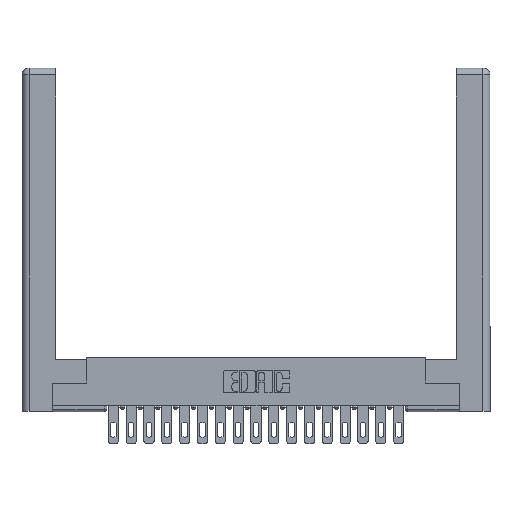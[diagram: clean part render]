
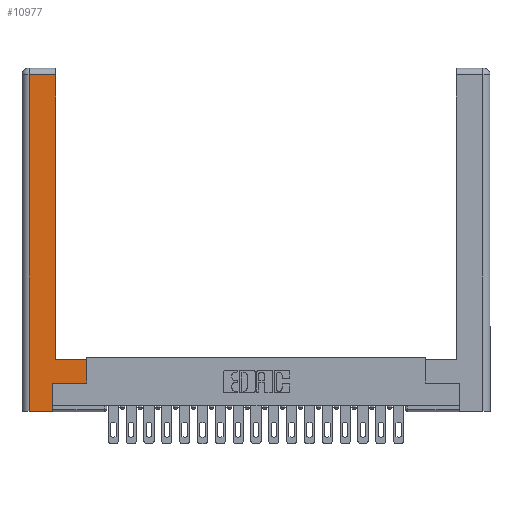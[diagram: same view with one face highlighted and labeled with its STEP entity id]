
A CAD part, top view. The second image highlights one B-rep face of the part: STEP entity #10977.
In plain terms, the highlighted planar face has unit normal (0, 0, 1).
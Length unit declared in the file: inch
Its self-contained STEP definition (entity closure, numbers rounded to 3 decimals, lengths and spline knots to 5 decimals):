
#130 = EDGE_CURVE ( 'NONE', #17198, #17549, #19335, .T. ) ;
#719 = PLANE ( 'NONE',  #18555 ) ;
#795 = ORIENTED_EDGE ( 'NONE', *, *, #10152, .T. ) ;
#1001 = ORIENTED_EDGE ( 'NONE', *, *, #14866, .T. ) ;
#1202 = ORIENTED_EDGE ( 'NONE', *, *, #11225, .T. ) ;
#1376 = CARTESIAN_POINT ( 'NONE',  ( 0.565, 0.245, 0. ) ) ;
#1582 = VERTEX_POINT ( 'NONE', #1671 ) ;
#1671 = CARTESIAN_POINT ( 'NONE',  ( 0.295, 2.94, 0. ) ) ;
#2708 = CARTESIAN_POINT ( 'NONE',  ( 0.265, 0.245, 0. ) ) ;
#3044 = EDGE_CURVE ( 'NONE', #17549, #8163, #11944, .T. ) ;
#3163 = EDGE_CURVE ( 'NONE', #14933, #9440, #14463, .T. ) ;
#3374 = ORIENTED_EDGE ( 'NONE', *, *, #130, .T. ) ;
#3509 = DIRECTION ( 'NONE',  ( 1., 0., 0. ) ) ;
#3822 = ORIENTED_EDGE ( 'NONE', *, *, #12952, .T. ) ;
#4591 = DIRECTION ( 'NONE',  ( 0., 1., 0. ) ) ;
#4656 = DIRECTION ( 'NONE',  ( 0., -1., 0. ) ) ;
#4859 = CARTESIAN_POINT ( 'NONE',  ( 0.0615, 0., 0. ) ) ;
#4863 = CARTESIAN_POINT ( 'NONE',  ( 0.265, 0., 0. ) ) ;
#5012 = CARTESIAN_POINT ( 'NONE',  ( 0.565, 0.45, 0. ) ) ;
#5196 = ORIENTED_EDGE ( 'NONE', *, *, #3044, .T. ) ;
#5393 = VECTOR ( 'NONE', #10994, 39.37008 ) ;
#5498 = CARTESIAN_POINT ( 'NONE',  ( 0., 0., 0. ) ) ;
#5504 = VECTOR ( 'NONE', #9365, 39.37008 ) ;
#6455 = EDGE_LOOP ( 'NONE', ( #795, #1202, #3822, #3374, #5196, #1001, #17080, #10570 ) ) ;
#6642 = DIRECTION ( 'NONE',  ( 0., 1., 0. ) ) ;
#6929 = DIRECTION ( 'NONE',  ( 0., 0., -1. ) ) ;
#7868 = CARTESIAN_POINT ( 'NONE',  ( 0.295, 3., 0. ) ) ;
#8163 = VERTEX_POINT ( 'NONE', #2708 ) ;
#9060 = CARTESIAN_POINT ( 'NONE',  ( 0.265, 0.245, 0. ) ) ;
#9365 = DIRECTION ( 'NONE',  ( 1., 0., 0. ) ) ;
#9440 = VERTEX_POINT ( 'NONE', #19036 ) ;
#9892 = EDGE_CURVE ( 'NONE', #9440, #15256, #20222, .T. ) ;
#10107 = CARTESIAN_POINT ( 'NONE',  ( 0.0615, 2.94, 0. ) ) ;
#10152 = EDGE_CURVE ( 'NONE', #15256, #1582, #18677, .T. ) ;
#10398 = VECTOR ( 'NONE', #3509, 39.37008 ) ;
#10570 = ORIENTED_EDGE ( 'NONE', *, *, #9892, .T. ) ;
#10977 = ADVANCED_FACE ( 'NONE', ( #11582 ), #719, .F. ) ;
#10994 = DIRECTION ( 'NONE',  ( -1., 0., 0. ) ) ;
#11125 = LINE ( 'NONE', #4859, #18955 ) ;
#11225 = EDGE_CURVE ( 'NONE', #1582, #20053, #15953, .T. ) ;
#11463 = CARTESIAN_POINT ( 'NONE',  ( 0.0615, 0., 0. ) ) ;
#11582 = FACE_OUTER_BOUND ( 'NONE', #6455, .T. ) ;
#11944 = LINE ( 'NONE', #9060, #19450 ) ;
#12004 = VECTOR ( 'NONE', #16057, 39.37008 ) ;
#12952 = EDGE_CURVE ( 'NONE', #20053, #17198, #11125, .T. ) ;
#13089 = VECTOR ( 'NONE', #6642, 39.37008 ) ;
#13216 = DIRECTION ( 'NONE',  ( -1., 0., 0. ) ) ;
#13477 = DIRECTION ( 'NONE',  ( 0., 1., 0. ) ) ;
#14275 = CARTESIAN_POINT ( 'NONE',  ( 0.565, 0.245, 0. ) ) ;
#14463 = LINE ( 'NONE', #5012, #13089 ) ;
#14707 = CARTESIAN_POINT ( 'NONE',  ( 0.0615, 2.94, 0. ) ) ;
#14866 = EDGE_CURVE ( 'NONE', #8163, #14933, #15520, .T. ) ;
#14933 = VERTEX_POINT ( 'NONE', #14275 ) ;
#15256 = VERTEX_POINT ( 'NONE', #19903 ) ;
#15520 = LINE ( 'NONE', #1376, #5504 ) ;
#15953 = LINE ( 'NONE', #14707, #12004 ) ;
#16057 = DIRECTION ( 'NONE',  ( -1., 0., 0. ) ) ;
#16344 = CARTESIAN_POINT ( 'NONE',  ( 0.265, 0., 0. ) ) ;
#17080 = ORIENTED_EDGE ( 'NONE', *, *, #3163, .T. ) ;
#17198 = VERTEX_POINT ( 'NONE', #11463 ) ;
#17222 = VECTOR ( 'NONE', #4591, 39.37008 ) ;
#17549 = VERTEX_POINT ( 'NONE', #4863 ) ;
#18555 = AXIS2_PLACEMENT_3D ( 'NONE', #5498, #6929, #13216 ) ;
#18677 = LINE ( 'NONE', #7868, #17222 ) ;
#18904 = CARTESIAN_POINT ( 'NONE',  ( 0.295, 0.45, 0. ) ) ;
#18955 = VECTOR ( 'NONE', #4656, 39.37008 ) ;
#19036 = CARTESIAN_POINT ( 'NONE',  ( 0.565, 0.45, 0. ) ) ;
#19335 = LINE ( 'NONE', #16344, #10398 ) ;
#19450 = VECTOR ( 'NONE', #13477, 39.37008 ) ;
#19903 = CARTESIAN_POINT ( 'NONE',  ( 0.295, 0.45, 0. ) ) ;
#20053 = VERTEX_POINT ( 'NONE', #10107 ) ;
#20222 = LINE ( 'NONE', #18904, #5393 ) ;
